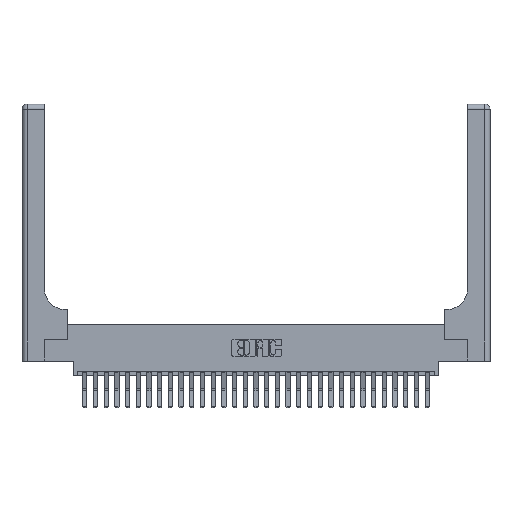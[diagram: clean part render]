
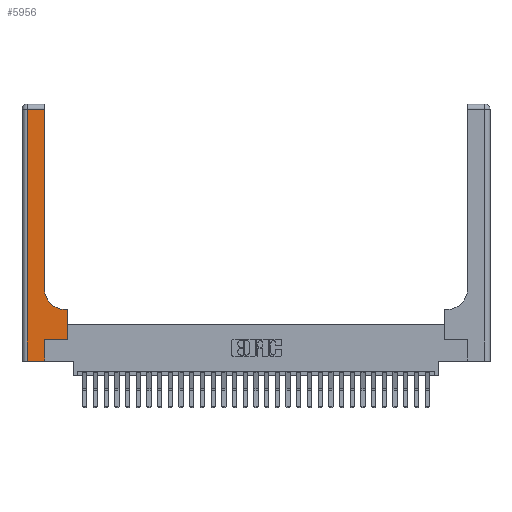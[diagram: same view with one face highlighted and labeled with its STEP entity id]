
A CAD part, top view. The second image highlights one B-rep face of the part: STEP entity #5956.
In plain terms, the highlighted planar face has unit normal (0, 0, 1).
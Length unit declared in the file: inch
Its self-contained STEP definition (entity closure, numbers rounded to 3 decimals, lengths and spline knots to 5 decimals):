
#619 = CIRCLE ( 'NONE', #16348, 0.25 ) ;
#686 = CARTESIAN_POINT ( 'NONE',  ( 0.51, 0.85, 0.37 ) ) ;
#1046 = EDGE_CURVE ( 'NONE', #23162, #19792, #7616, .T. ) ;
#1796 = CARTESIAN_POINT ( 'NONE',  ( 0.26, 3., 0.37 ) ) ;
#1921 = CARTESIAN_POINT ( 'NONE',  ( 0., 3., 0.37 ) ) ;
#3603 = AXIS2_PLACEMENT_3D ( 'NONE', #1921, #11019, #8597 ) ;
#3742 = DIRECTION ( 'NONE',  ( -1., 0., 0. ) ) ;
#4811 = VERTEX_POINT ( 'NONE', #11827 ) ;
#4898 = ORIENTED_EDGE ( 'NONE', *, *, #7385, .T. ) ;
#4938 = EDGE_CURVE ( 'NONE', #23622, #4811, #619, .T. ) ;
#5911 = CARTESIAN_POINT ( 'NONE',  ( 0., 2.94, 0.37 ) ) ;
#5956 = ADVANCED_FACE ( 'NONE', ( #20142 ), #28413, .F. ) ;
#7165 = CARTESIAN_POINT ( 'NONE',  ( 0.26, 2.94, 0.37 ) ) ;
#7238 = DIRECTION ( 'NONE',  ( 1., 0., 0. ) ) ;
#7363 = CARTESIAN_POINT ( 'NONE',  ( 0.265, 0., 0.37 ) ) ;
#7385 = EDGE_CURVE ( 'NONE', #18555, #13333, #23315, .T. ) ;
#7616 = LINE ( 'NONE', #25262, #28449 ) ;
#8535 = VERTEX_POINT ( 'NONE', #13353 ) ;
#8597 = DIRECTION ( 'NONE',  ( -1., 0., 0. ) ) ;
#10023 = DIRECTION ( 'NONE',  ( 0., -1., 0. ) ) ;
#10119 = ORIENTED_EDGE ( 'NONE', *, *, #24300, .T. ) ;
#10925 = EDGE_LOOP ( 'NONE', ( #24356, #19743, #4898, #22819, #11165, #19927, #10119, #16191, #16293 ) ) ;
#11019 = DIRECTION ( 'NONE',  ( 0., 0., -1. ) ) ;
#11165 = ORIENTED_EDGE ( 'NONE', *, *, #1046, .T. ) ;
#11827 = CARTESIAN_POINT ( 'NONE',  ( 0.26, 0.85, 0.37 ) ) ;
#11997 = LINE ( 'NONE', #16505, #21579 ) ;
#12641 = EDGE_CURVE ( 'NONE', #4811, #24395, #17573, .T. ) ;
#12969 = DIRECTION ( 'NONE',  ( 0., 1., 0. ) ) ;
#13202 = EDGE_CURVE ( 'NONE', #19792, #24905, #15920, .T. ) ;
#13333 = VERTEX_POINT ( 'NONE', #21228 ) ;
#13353 = CARTESIAN_POINT ( 'NONE',  ( 0.528, 0.6, 0.37 ) ) ;
#13790 = VECTOR ( 'NONE', #3742, 39.37008 ) ;
#15089 = EDGE_CURVE ( 'NONE', #8535, #23622, #23396, .T. ) ;
#15141 = CARTESIAN_POINT ( 'NONE',  ( 0.528, 0.25, 0.37 ) ) ;
#15272 = LINE ( 'NONE', #15141, #17161 ) ;
#15920 = LINE ( 'NONE', #18093, #20450 ) ;
#16179 = DIRECTION ( 'NONE',  ( 0., 0., -1. ) ) ;
#16191 = ORIENTED_EDGE ( 'NONE', *, *, #15089, .T. ) ;
#16293 = ORIENTED_EDGE ( 'NONE', *, *, #4938, .T. ) ;
#16348 = AXIS2_PLACEMENT_3D ( 'NONE', #686, #16179, #28185 ) ;
#16505 = CARTESIAN_POINT ( 'NONE',  ( 0., 0., 0.37 ) ) ;
#17161 = VECTOR ( 'NONE', #12969, 39.37008 ) ;
#17536 = CARTESIAN_POINT ( 'NONE',  ( 0.51, 0.6, 0.37 ) ) ;
#17573 = LINE ( 'NONE', #1796, #28366 ) ;
#17937 = EDGE_CURVE ( 'NONE', #13333, #23162, #11997, .T. ) ;
#18004 = CARTESIAN_POINT ( 'NONE',  ( 0.265, 0.25, 0.37 ) ) ;
#18093 = CARTESIAN_POINT ( 'NONE',  ( 0.265, 0.25, 0.37 ) ) ;
#18555 = VERTEX_POINT ( 'NONE', #19217 ) ;
#18713 = CARTESIAN_POINT ( 'NONE',  ( 0.06, 3., 0.37 ) ) ;
#18760 = DIRECTION ( 'NONE',  ( 0., 1., 0. ) ) ;
#19077 = LINE ( 'NONE', #5911, #13790 ) ;
#19217 = CARTESIAN_POINT ( 'NONE',  ( 0.06, 2.94, 0.37 ) ) ;
#19304 = EDGE_CURVE ( 'NONE', #24395, #18555, #19077, .T. ) ;
#19396 = CARTESIAN_POINT ( 'NONE',  ( 0.528, 0.25, 0.37 ) ) ;
#19743 = ORIENTED_EDGE ( 'NONE', *, *, #19304, .T. ) ;
#19792 = VERTEX_POINT ( 'NONE', #18004 ) ;
#19927 = ORIENTED_EDGE ( 'NONE', *, *, #13202, .T. ) ;
#20142 = FACE_OUTER_BOUND ( 'NONE', #10925, .T. ) ;
#20450 = VECTOR ( 'NONE', #7238, 39.37008 ) ;
#20687 = DIRECTION ( 'NONE',  ( 1., 0., 0. ) ) ;
#21228 = CARTESIAN_POINT ( 'NONE',  ( 0.06, 0., 0.37 ) ) ;
#21579 = VECTOR ( 'NONE', #20687, 39.37008 ) ;
#22819 = ORIENTED_EDGE ( 'NONE', *, *, #17937, .T. ) ;
#23162 = VERTEX_POINT ( 'NONE', #7363 ) ;
#23315 = LINE ( 'NONE', #18713, #24019 ) ;
#23396 = LINE ( 'NONE', #27603, #27001 ) ;
#23622 = VERTEX_POINT ( 'NONE', #17536 ) ;
#24019 = VECTOR ( 'NONE', #10023, 39.37008 ) ;
#24300 = EDGE_CURVE ( 'NONE', #24905, #8535, #15272, .T. ) ;
#24356 = ORIENTED_EDGE ( 'NONE', *, *, #12641, .T. ) ;
#24395 = VERTEX_POINT ( 'NONE', #7165 ) ;
#24905 = VERTEX_POINT ( 'NONE', #19396 ) ;
#25150 = DIRECTION ( 'NONE',  ( -1., 0., 0. ) ) ;
#25262 = CARTESIAN_POINT ( 'NONE',  ( 0.265, 0., 0.37 ) ) ;
#26388 = DIRECTION ( 'NONE',  ( 0., 1., 0. ) ) ;
#27001 = VECTOR ( 'NONE', #25150, 39.37008 ) ;
#27603 = CARTESIAN_POINT ( 'NONE',  ( 0.26, 0.6, 0.37 ) ) ;
#28185 = DIRECTION ( 'NONE',  ( 1., 0., 0. ) ) ;
#28366 = VECTOR ( 'NONE', #26388, 39.37008 ) ;
#28413 = PLANE ( 'NONE',  #3603 ) ;
#28449 = VECTOR ( 'NONE', #18760, 39.37008 ) ;
